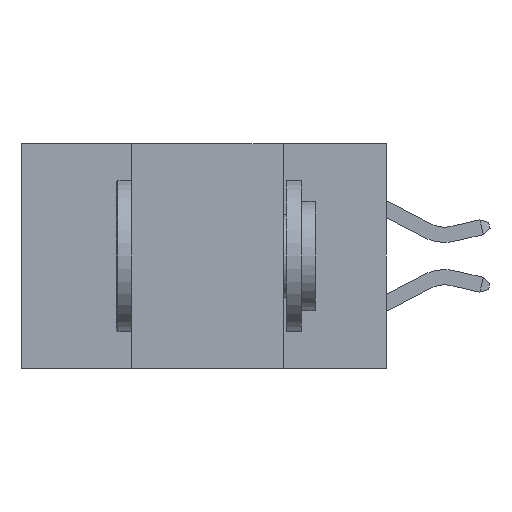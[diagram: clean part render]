
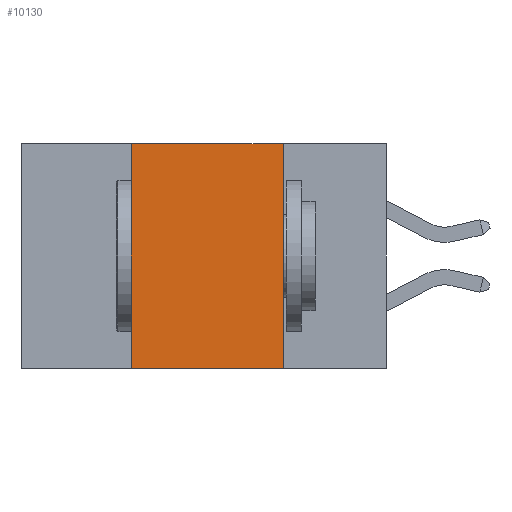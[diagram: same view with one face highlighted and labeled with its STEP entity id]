
A CAD part, left-side view. The second image highlights one B-rep face of the part: STEP entity #10130.
In plain terms, the highlighted planar face has unit normal (-1, 0, 0).
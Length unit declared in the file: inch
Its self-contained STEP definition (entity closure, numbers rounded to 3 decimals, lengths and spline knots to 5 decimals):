
#424 = VERTEX_POINT ( 'NONE', #1680 ) ;
#828 = ORIENTED_EDGE ( 'NONE', *, *, #8826, .T. ) ;
#1336 = VERTEX_POINT ( 'NONE', #6053 ) ;
#1584 = ORIENTED_EDGE ( 'NONE', *, *, #7521, .F. ) ;
#1638 = LINE ( 'NONE', #7042, #5985 ) ;
#1680 = CARTESIAN_POINT ( 'NONE',  ( 0., 0.17, 0. ) ) ;
#2371 = EDGE_LOOP ( 'NONE', ( #1584, #10787, #7950, #828 ) ) ;
#2467 = DIRECTION ( 'NONE',  ( 0., 0., -1. ) ) ;
#3516 = DIRECTION ( 'NONE',  ( 1., 0., 0. ) ) ;
#3592 = VECTOR ( 'NONE', #4281, 39.37008 ) ;
#4220 = LINE ( 'NONE', #9817, #3592 ) ;
#4281 = DIRECTION ( 'NONE',  ( 0., -1., 0. ) ) ;
#4347 = EDGE_CURVE ( 'NONE', #10855, #9330, #4926, .T. ) ;
#4421 = CARTESIAN_POINT ( 'NONE',  ( 0., 0.6, 0. ) ) ;
#4446 = DIRECTION ( 'NONE',  ( 0., -1., 0. ) ) ;
#4493 = DIRECTION ( 'NONE',  ( 0., 0., -1. ) ) ;
#4577 = EDGE_CURVE ( 'NONE', #9330, #424, #9189, .T. ) ;
#4604 = VECTOR ( 'NONE', #4446, 39.37008 ) ;
#4926 = LINE ( 'NONE', #5642, #6886 ) ;
#5424 = CARTESIAN_POINT ( 'NONE',  ( 0., 0.42, 0. ) ) ;
#5642 = CARTESIAN_POINT ( 'NONE',  ( 0., 0.42, -0.37 ) ) ;
#5985 = VECTOR ( 'NONE', #4493, 39.37008 ) ;
#6053 = CARTESIAN_POINT ( 'NONE',  ( 0., 0.17, -0.37 ) ) ;
#6186 = CARTESIAN_POINT ( 'NONE',  ( 0., 0.6, 0. ) ) ;
#6596 = DIRECTION ( 'NONE',  ( 0., 0., 1. ) ) ;
#6886 = VECTOR ( 'NONE', #6596, 39.37008 ) ;
#7042 = CARTESIAN_POINT ( 'NONE',  ( 0., 0.17, -0.37 ) ) ;
#7173 = FACE_OUTER_BOUND ( 'NONE', #2371, .T. ) ;
#7521 = EDGE_CURVE ( 'NONE', #424, #1336, #1638, .T. ) ;
#7950 = ORIENTED_EDGE ( 'NONE', *, *, #4347, .F. ) ;
#8826 = EDGE_CURVE ( 'NONE', #10855, #1336, #4220, .T. ) ;
#9189 = LINE ( 'NONE', #4421, #4604 ) ;
#9265 = CARTESIAN_POINT ( 'NONE',  ( 0., 0.42, -0.37 ) ) ;
#9330 = VERTEX_POINT ( 'NONE', #5424 ) ;
#9817 = CARTESIAN_POINT ( 'NONE',  ( 0., 0.6, -0.37 ) ) ;
#10130 = ADVANCED_FACE ( 'NONE', ( #7173 ), #10648, .F. ) ;
#10648 = PLANE ( 'NONE',  #11505 ) ;
#10787 = ORIENTED_EDGE ( 'NONE', *, *, #4577, .F. ) ;
#10855 = VERTEX_POINT ( 'NONE', #9265 ) ;
#11505 = AXIS2_PLACEMENT_3D ( 'NONE', #6186, #3516, #2467 ) ;
